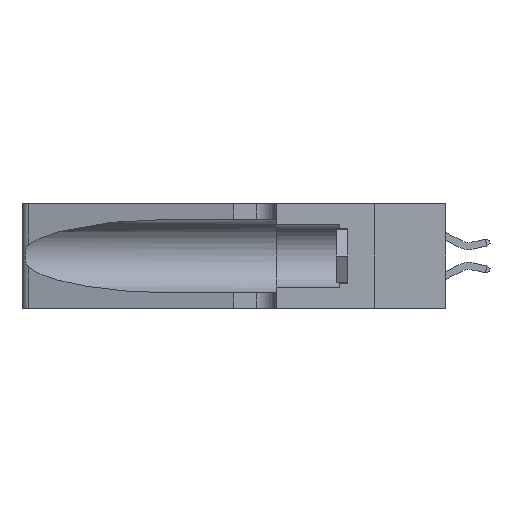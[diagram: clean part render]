
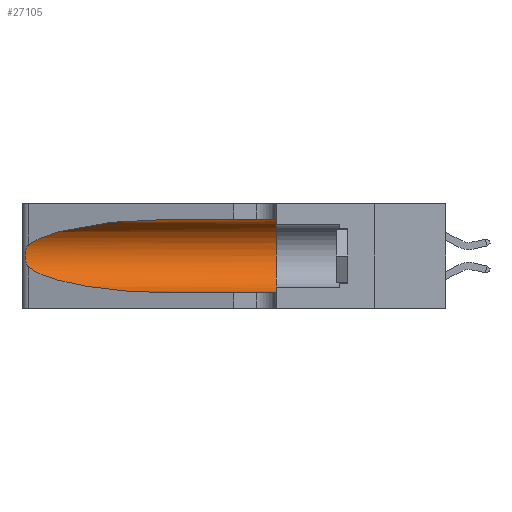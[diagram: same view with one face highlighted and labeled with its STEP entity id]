
A CAD part, left-side view. The second image highlights one B-rep face of the part: STEP entity #27105.
In plain terms, the highlighted cylindrical face has radius 3.308 mm (diameter 6.617 mm), a partial arc.
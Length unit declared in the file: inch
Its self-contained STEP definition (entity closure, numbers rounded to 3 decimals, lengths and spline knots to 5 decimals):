
#144 = CARTESIAN_POINT ( 'NONE',  ( 0.18966, 0.96281, 0.31525 ) ) ;
#1039 = VERTEX_POINT ( 'NONE', #4787 ) ;
#1536 = LINE ( 'NONE', #18418, #23268 ) ;
#1548 = CARTESIAN_POINT ( 'NONE',  ( 0.25555, 1.22993, 0.14849 ) ) ;
#1590 = VERTEX_POINT ( 'NONE', #18641 ) ;
#3019 = CARTESIAN_POINT ( 'NONE',  ( 0.1305, 0.72297, 0.31525 ) ) ;
#4787 = CARTESIAN_POINT ( 'NONE',  ( 0.25487, 1.22718, 0.14631 ) ) ;
#5605 = CARTESIAN_POINT ( 'NONE',  ( 0.2373, 1.15595, 0.08982 ) ) ;
#6040 = CARTESIAN_POINT ( 'NONE',  ( 0.25487, 1.22718, 0.22369 ) ) ;
#6528 = LINE ( 'NONE', #33188, #25445 ) ;
#7238 = CARTESIAN_POINT ( 'NONE',  ( 0.25787, 1.23484, 0.2124 ) ) ;
#8572 =( BOUNDED_CURVE ( )  B_SPLINE_CURVE ( 3, ( #25293, #5605, #14085, #33778 ),
 .UNSPECIFIED., .F., .T. ) 
 B_SPLINE_CURVE_WITH_KNOTS ( ( 4, 4 ),
 ( 3.44316, 4.71239 ),
 .UNSPECIFIED. ) 
 CURVE ( )  GEOMETRIC_REPRESENTATION_ITEM ( )  RATIONAL_B_SPLINE_CURVE ( ( 1., 0.87, 0.87, 1. ) ) 
 REPRESENTATION_ITEM ( '' )  );
#10053 = CARTESIAN_POINT ( 'NONE',  ( 0.26018, 1.23835, 0.19895 ) ) ;
#10346 = EDGE_CURVE ( 'NONE', #18507, #33333, #1536, .T. ) ;
#10514 = EDGE_CURVE ( 'NONE', #13121, #14956, #6528, .T. ) ;
#10640 = EDGE_CURVE ( 'NONE', #14956, #33333, #21011, .T. ) ;
#11560 = CARTESIAN_POINT ( 'NONE',  ( 0.1305, 0.72297, 0.31525 ) ) ;
#12032 = EDGE_CURVE ( 'NONE', #13121, #1590, #28187, .T. ) ;
#12881 = CARTESIAN_POINT ( 'NONE',  ( 0.26075, 1.23896, 0.178 ) ) ;
#13121 = VERTEX_POINT ( 'NONE', #3019 ) ;
#13390 = ORIENTED_EDGE ( 'NONE', *, *, #10640, .F. ) ;
#14050 = EDGE_CURVE ( 'NONE', #1590, #1039, #15111, .T. ) ;
#14085 = CARTESIAN_POINT ( 'NONE',  ( 0.18966, 0.96281, 0.05475 ) ) ;
#14225 = CARTESIAN_POINT ( 'NONE',  ( 0.1305, 0.35, 0.185 ) ) ;
#14956 = VERTEX_POINT ( 'NONE', #22409 ) ;
#15058 = CARTESIAN_POINT ( 'NONE',  ( 0.1305, 1.61858, 0.185 ) ) ;
#15111 = B_SPLINE_CURVE_WITH_KNOTS ( 'NONE', 3,
 ( #35278, #26808, #24078, #7238, #26934, #10053, #29760, #12881, #32592, #15707, #35391, #18520, #1548, #21353 ),
 .UNSPECIFIED., .F., .F.,
 ( 4, 2, 2, 2, 2, 2, 4 ),
 ( 0., 0.00027, 0.00053, 0.00107, 0.0016, 0.00187, 0.00214 ),
 .UNSPECIFIED. ) ;
#15610 = DIRECTION ( 'NONE',  ( 0., -1., 0. ) ) ;
#15707 = CARTESIAN_POINT ( 'NONE',  ( 0.25856, 1.23593, 0.16098 ) ) ;
#16325 = CYLINDRICAL_SURFACE ( 'NONE', #29040, 0.13025 ) ;
#17053 = DIRECTION ( 'NONE',  ( 0., 0., 1. ) ) ;
#17285 = EDGE_CURVE ( 'NONE', #1039, #18507, #8572, .T. ) ;
#17312 = AXIS2_PLACEMENT_3D ( 'NONE', #14225, #33924, #17053 ) ;
#17869 = DIRECTION ( 'NONE',  ( 0., -1., 0. ) ) ;
#18418 = CARTESIAN_POINT ( 'NONE',  ( 0.1305, 1.61858, 0.05475 ) ) ;
#18507 = VERTEX_POINT ( 'NONE', #25227 ) ;
#18520 = CARTESIAN_POINT ( 'NONE',  ( 0.25639, 1.23186, 0.15144 ) ) ;
#18641 = CARTESIAN_POINT ( 'NONE',  ( 0.25487, 1.22718, 0.22369 ) ) ;
#19304 = ORIENTED_EDGE ( 'NONE', *, *, #14050, .T. ) ;
#20690 = DIRECTION ( 'NONE',  ( 0., 0., -1. ) ) ;
#21011 = CIRCLE ( 'NONE', #17312, 0.13025 ) ;
#21353 = CARTESIAN_POINT ( 'NONE',  ( 0.25487, 1.22718, 0.14631 ) ) ;
#21856 = DIRECTION ( 'NONE',  ( 0., -1., 0. ) ) ;
#22409 = CARTESIAN_POINT ( 'NONE',  ( 0.1305, 0.35, 0.31525 ) ) ;
#22887 = CARTESIAN_POINT ( 'NONE',  ( 0.2373, 1.15595, 0.28018 ) ) ;
#23268 = VECTOR ( 'NONE', #15610, 39.37008 ) ;
#23586 = ORIENTED_EDGE ( 'NONE', *, *, #10514, .F. ) ;
#23817 = FACE_OUTER_BOUND ( 'NONE', #33405, .T. ) ;
#24078 = CARTESIAN_POINT ( 'NONE',  ( 0.25639, 1.23184, 0.21858 ) ) ;
#25227 = CARTESIAN_POINT ( 'NONE',  ( 0.1305, 0.72297, 0.05475 ) ) ;
#25293 = CARTESIAN_POINT ( 'NONE',  ( 0.25487, 1.22718, 0.14631 ) ) ;
#25445 = VECTOR ( 'NONE', #21856, 39.37008 ) ;
#26057 = ORIENTED_EDGE ( 'NONE', *, *, #10346, .T. ) ;
#26808 = CARTESIAN_POINT ( 'NONE',  ( 0.25555, 1.22994, 0.2215 ) ) ;
#26934 = CARTESIAN_POINT ( 'NONE',  ( 0.25854, 1.2359, 0.20912 ) ) ;
#27105 = ADVANCED_FACE ( 'NONE', ( #23817 ), #16325, .F. ) ;
#28187 =( BOUNDED_CURVE ( )  B_SPLINE_CURVE ( 3, ( #11560, #144, #22887, #6040 ),
 .UNSPECIFIED., .F., .F. ) 
 B_SPLINE_CURVE_WITH_KNOTS ( ( 4, 4 ),
 ( 1.5708, 2.84003 ),
 .UNSPECIFIED. ) 
 CURVE ( )  GEOMETRIC_REPRESENTATION_ITEM ( )  RATIONAL_B_SPLINE_CURVE ( ( 1., 0.87, 0.87, 1. ) ) 
 REPRESENTATION_ITEM ( '' )  );
#28458 = ORIENTED_EDGE ( 'NONE', *, *, #12032, .T. ) ;
#29039 = ORIENTED_EDGE ( 'NONE', *, *, #17285, .T. ) ;
#29040 = AXIS2_PLACEMENT_3D ( 'NONE', #15058, #17869, #20690 ) ;
#29760 = CARTESIAN_POINT ( 'NONE',  ( 0.26075, 1.23896, 0.19203 ) ) ;
#31625 = CARTESIAN_POINT ( 'NONE',  ( 0.1305, 0.35, 0.05475 ) ) ;
#32592 = CARTESIAN_POINT ( 'NONE',  ( 0.26017, 1.23833, 0.17102 ) ) ;
#33188 = CARTESIAN_POINT ( 'NONE',  ( 0.1305, 1.61858, 0.31525 ) ) ;
#33333 = VERTEX_POINT ( 'NONE', #31625 ) ;
#33405 = EDGE_LOOP ( 'NONE', ( #28458, #19304, #29039, #26057, #13390, #23586 ) ) ;
#33778 = CARTESIAN_POINT ( 'NONE',  ( 0.1305, 0.72297, 0.05475 ) ) ;
#33924 = DIRECTION ( 'NONE',  ( 0., 1., 0. ) ) ;
#35278 = CARTESIAN_POINT ( 'NONE',  ( 0.25487, 1.22718, 0.22369 ) ) ;
#35391 = CARTESIAN_POINT ( 'NONE',  ( 0.25789, 1.23486, 0.15765 ) ) ;
